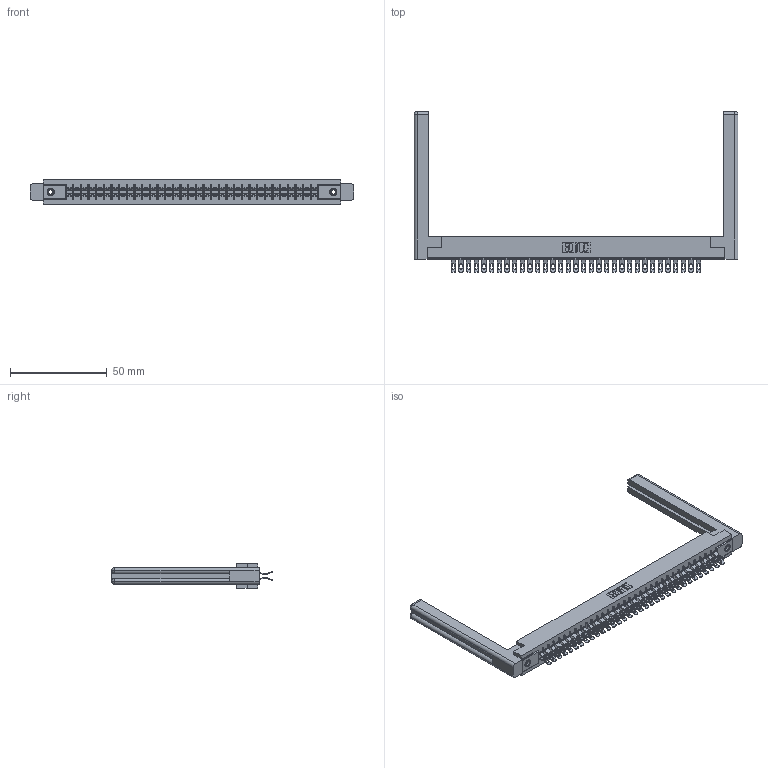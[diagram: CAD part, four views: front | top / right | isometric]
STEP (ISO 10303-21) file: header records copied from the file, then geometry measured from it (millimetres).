
FILE_DESCRIPTION (( 'STEP AP203' ), '1' );
FILE_NAME ('315-066-555-258.STEP', '2019-09-10T20:56:22', ( '' ), ( '' ), 'SwSTEP 2.0', 'SolidWorks 2016', '' );
FILE_SCHEMA (( 'CONFIG_CONTROL_DESIGN' ));
Length unit declared in the file: inch
Products named in the file (5): 345-250-001_345-250-001-102; 315-066-555-258; 307-220-058; 305 Part_.156 Dia; 305-290-001_555
Assembly tree (71 placements, depth 2):
  315-066-555-258
    305 Part_.156 Dia
    305-290-001_555  x66
    345-250-001_345-250-001-102  x2
    307-220-058  x2
Bounding box: 167.39 x 83.06 x 12.7 mm (x, y, z)
Volume: 24763.2 mm3; surface area: 28286.2 mm2
Topology: 71 solids, 71 shells, 4614 faces, 13705 edges, 8946 vertices
Faces by surface type: plane 2264, cylinder 2194, sphere 132, cone 12, torus 12
Entity records: 40083 total; most frequent: CARTESIAN_POINT 6666, ORIENTED_EDGE 6548, DIRECTION 6412, EDGE_CURVE 3274, LINE 2608, VECTOR 2608, VERTEX_POINT 2086, AXIS2_PLACEMENT_3D 1902
